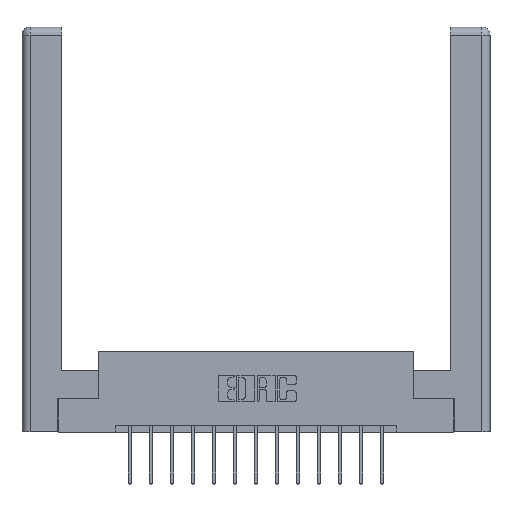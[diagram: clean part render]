
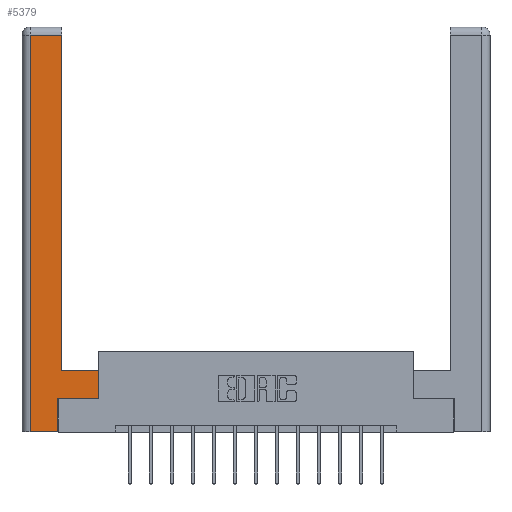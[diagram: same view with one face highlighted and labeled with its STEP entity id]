
A CAD part, top view. The second image highlights one B-rep face of the part: STEP entity #5379.
In plain terms, the highlighted planar face has unit normal (0, 0, 1).
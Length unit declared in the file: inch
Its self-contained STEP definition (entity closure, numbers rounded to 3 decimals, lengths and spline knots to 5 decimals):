
#5 = AXIS2_PLACEMENT_3D ( 'NONE', #6963, #5726, #10763 ) ;
#115 = EDGE_CURVE ( 'NONE', #3163, #10332, #10133, .T. ) ;
#192 = DIRECTION ( 'NONE',  ( 1., 0., 0. ) ) ;
#204 = CARTESIAN_POINT ( 'NONE',  ( 0.295, 2.94, 0. ) ) ;
#503 = ORIENTED_EDGE ( 'NONE', *, *, #8661, .T. ) ;
#890 = CARTESIAN_POINT ( 'NONE',  ( 0.265, 0.245, 0. ) ) ;
#1371 = DIRECTION ( 'NONE',  ( -1., 0., 0. ) ) ;
#2072 = VECTOR ( 'NONE', #1371, 39.37008 ) ;
#2439 = DIRECTION ( 'NONE',  ( 0., -1., 0. ) ) ;
#2601 = VERTEX_POINT ( 'NONE', #204 ) ;
#2967 = CARTESIAN_POINT ( 'NONE',  ( 0.565, 0.45, 0. ) ) ;
#3163 = VERTEX_POINT ( 'NONE', #4769 ) ;
#3346 = VECTOR ( 'NONE', #5721, 39.37008 ) ;
#3527 = VECTOR ( 'NONE', #10083, 39.37008 ) ;
#4295 = ORIENTED_EDGE ( 'NONE', *, *, #8100, .T. ) ;
#4416 = ORIENTED_EDGE ( 'NONE', *, *, #11071, .T. ) ;
#4769 = CARTESIAN_POINT ( 'NONE',  ( 0.0615, 0., 0. ) ) ;
#5309 = CARTESIAN_POINT ( 'NONE',  ( 0.265, 0.245, 0. ) ) ;
#5379 = ADVANCED_FACE ( 'NONE', ( #14967 ), #9346, .F. ) ;
#5721 = DIRECTION ( 'NONE',  ( 0., 1., 0. ) ) ;
#5726 = DIRECTION ( 'NONE',  ( 0., 0., -1. ) ) ;
#5787 = VECTOR ( 'NONE', #14272, 39.37008 ) ;
#6256 = CARTESIAN_POINT ( 'NONE',  ( 0.0615, 2.94, 0. ) ) ;
#6345 = CARTESIAN_POINT ( 'NONE',  ( 0.295, 0.45, 0. ) ) ;
#6383 = LINE ( 'NONE', #15489, #13531 ) ;
#6455 = VECTOR ( 'NONE', #11705, 39.37008 ) ;
#6497 = CARTESIAN_POINT ( 'NONE',  ( 0.265, 0., 0. ) ) ;
#6537 = VERTEX_POINT ( 'NONE', #14728 ) ;
#6782 = VECTOR ( 'NONE', #192, 39.37008 ) ;
#6963 = CARTESIAN_POINT ( 'NONE',  ( 0., 0., 0. ) ) ;
#7148 = LINE ( 'NONE', #10917, #3346 ) ;
#7691 = CARTESIAN_POINT ( 'NONE',  ( 0.265, 0., 0. ) ) ;
#7862 = DIRECTION ( 'NONE',  ( 1., 0., 0. ) ) ;
#8030 = EDGE_LOOP ( 'NONE', ( #14539, #12689, #13072, #15733, #4295, #4416, #11447, #503 ) ) ;
#8100 = EDGE_CURVE ( 'NONE', #10332, #14863, #8846, .T. ) ;
#8661 = EDGE_CURVE ( 'NONE', #15366, #11213, #15809, .T. ) ;
#8846 = LINE ( 'NONE', #5309, #6455 ) ;
#9346 = PLANE ( 'NONE',  #5 ) ;
#10083 = DIRECTION ( 'NONE',  ( -1., 0., 0. ) ) ;
#10133 = LINE ( 'NONE', #6497, #6782 ) ;
#10279 = VERTEX_POINT ( 'NONE', #12690 ) ;
#10332 = VERTEX_POINT ( 'NONE', #7691 ) ;
#10763 = DIRECTION ( 'NONE',  ( -1., 0., 0. ) ) ;
#10917 = CARTESIAN_POINT ( 'NONE',  ( 0.565, 0.45, 0. ) ) ;
#11071 = EDGE_CURVE ( 'NONE', #14863, #6537, #6383, .T. ) ;
#11213 = VERTEX_POINT ( 'NONE', #6345 ) ;
#11367 = CARTESIAN_POINT ( 'NONE',  ( 0.0615, 0., 0. ) ) ;
#11447 = ORIENTED_EDGE ( 'NONE', *, *, #11756, .T. ) ;
#11463 = CARTESIAN_POINT ( 'NONE',  ( 0.295, 0.45, 0. ) ) ;
#11705 = DIRECTION ( 'NONE',  ( 0., 1., 0. ) ) ;
#11756 = EDGE_CURVE ( 'NONE', #6537, #15366, #7148, .T. ) ;
#11990 = EDGE_CURVE ( 'NONE', #2601, #10279, #14099, .T. ) ;
#12650 = EDGE_CURVE ( 'NONE', #11213, #2601, #12773, .T. ) ;
#12689 = ORIENTED_EDGE ( 'NONE', *, *, #11990, .T. ) ;
#12690 = CARTESIAN_POINT ( 'NONE',  ( 0.0615, 2.94, 0. ) ) ;
#12773 = LINE ( 'NONE', #13096, #5787 ) ;
#13072 = ORIENTED_EDGE ( 'NONE', *, *, #15508, .T. ) ;
#13096 = CARTESIAN_POINT ( 'NONE',  ( 0.295, 3., 0. ) ) ;
#13531 = VECTOR ( 'NONE', #7862, 39.37008 ) ;
#13925 = LINE ( 'NONE', #11367, #14925 ) ;
#14099 = LINE ( 'NONE', #6256, #3527 ) ;
#14272 = DIRECTION ( 'NONE',  ( 0., 1., 0. ) ) ;
#14539 = ORIENTED_EDGE ( 'NONE', *, *, #12650, .T. ) ;
#14728 = CARTESIAN_POINT ( 'NONE',  ( 0.565, 0.245, 0. ) ) ;
#14863 = VERTEX_POINT ( 'NONE', #890 ) ;
#14925 = VECTOR ( 'NONE', #2439, 39.37008 ) ;
#14967 = FACE_OUTER_BOUND ( 'NONE', #8030, .T. ) ;
#15366 = VERTEX_POINT ( 'NONE', #2967 ) ;
#15489 = CARTESIAN_POINT ( 'NONE',  ( 0.565, 0.245, 0. ) ) ;
#15508 = EDGE_CURVE ( 'NONE', #10279, #3163, #13925, .T. ) ;
#15733 = ORIENTED_EDGE ( 'NONE', *, *, #115, .T. ) ;
#15809 = LINE ( 'NONE', #11463, #2072 ) ;
